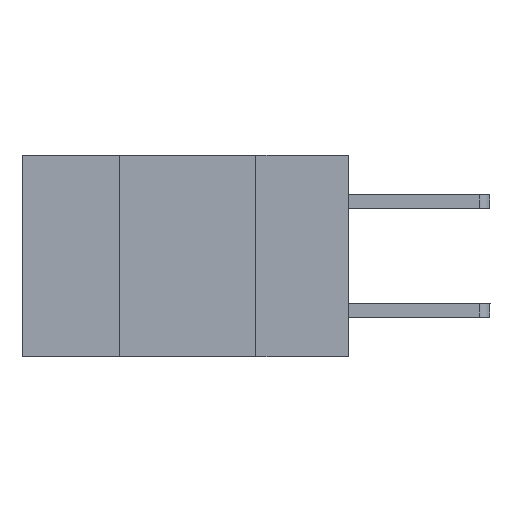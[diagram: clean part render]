
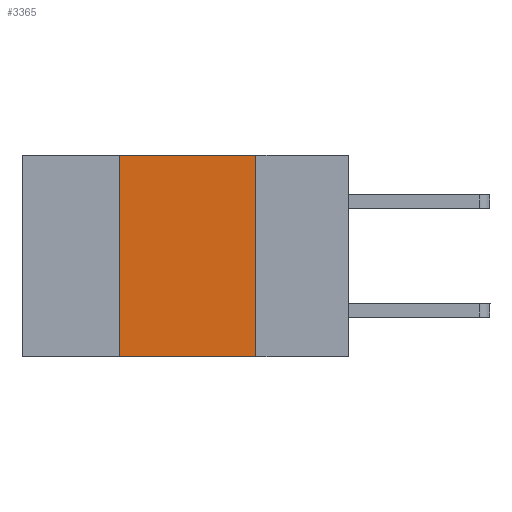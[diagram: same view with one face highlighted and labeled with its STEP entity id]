
A CAD part, left-side view. The second image highlights one B-rep face of the part: STEP entity #3365.
In plain terms, the highlighted planar face has unit normal (-1, 0, 0).
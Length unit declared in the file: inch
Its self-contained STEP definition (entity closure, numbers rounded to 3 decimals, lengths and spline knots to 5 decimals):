
#161 = VERTEX_POINT ( 'NONE', #2700 ) ;
#421 = ORIENTED_EDGE ( 'NONE', *, *, #1642, .T. ) ;
#592 = AXIS2_PLACEMENT_3D ( 'NONE', #3027, #1663, #1645 ) ;
#651 = EDGE_CURVE ( 'NONE', #161, #4681, #4739, .T. ) ;
#888 = EDGE_CURVE ( 'NONE', #4681, #3417, #6702, .T. ) ;
#996 = EDGE_CURVE ( 'NONE', #3417, #4597, #3637, .T. ) ;
#1642 = EDGE_CURVE ( 'NONE', #161, #4597, #7716, .T. ) ;
#1645 = DIRECTION ( 'NONE',  ( 0., 0., -1. ) ) ;
#1663 = DIRECTION ( 'NONE',  ( 1., 0., 0. ) ) ;
#1760 = PLANE ( 'NONE',  #592 ) ;
#2589 = ORIENTED_EDGE ( 'NONE', *, *, #888, .F. ) ;
#2700 = CARTESIAN_POINT ( 'NONE',  ( 0., 0.42, -0.37 ) ) ;
#3027 = CARTESIAN_POINT ( 'NONE',  ( 0., 0.6, 0. ) ) ;
#3066 = DIRECTION ( 'NONE',  ( 0., -1., 0. ) ) ;
#3162 = DIRECTION ( 'NONE',  ( 0., -1., 0. ) ) ;
#3365 = ADVANCED_FACE ( 'NONE', ( #3757 ), #1760, .F. ) ;
#3417 = VERTEX_POINT ( 'NONE', #8166 ) ;
#3637 = LINE ( 'NONE', #5191, #5474 ) ;
#3757 = FACE_OUTER_BOUND ( 'NONE', #5727, .T. ) ;
#4597 = VERTEX_POINT ( 'NONE', #7343 ) ;
#4681 = VERTEX_POINT ( 'NONE', #6248 ) ;
#4739 = LINE ( 'NONE', #7627, #9024 ) ;
#4929 = VECTOR ( 'NONE', #3162, 39.37008 ) ;
#5191 = CARTESIAN_POINT ( 'NONE',  ( 0., 0.17, -0.37 ) ) ;
#5474 = VECTOR ( 'NONE', #8913, 39.37008 ) ;
#5727 = EDGE_LOOP ( 'NONE', ( #6177, #2589, #6173, #421 ) ) ;
#5986 = VECTOR ( 'NONE', #3066, 39.37008 ) ;
#6173 = ORIENTED_EDGE ( 'NONE', *, *, #651, .F. ) ;
#6177 = ORIENTED_EDGE ( 'NONE', *, *, #996, .F. ) ;
#6248 = CARTESIAN_POINT ( 'NONE',  ( 0., 0.42, 0. ) ) ;
#6702 = LINE ( 'NONE', #7554, #4929 ) ;
#6846 = CARTESIAN_POINT ( 'NONE',  ( 0., 0.6, -0.37 ) ) ;
#7343 = CARTESIAN_POINT ( 'NONE',  ( 0., 0.17, -0.37 ) ) ;
#7554 = CARTESIAN_POINT ( 'NONE',  ( 0., 0.6, 0. ) ) ;
#7627 = CARTESIAN_POINT ( 'NONE',  ( 0., 0.42, -0.37 ) ) ;
#7716 = LINE ( 'NONE', #6846, #5986 ) ;
#8043 = DIRECTION ( 'NONE',  ( 0., 0., 1. ) ) ;
#8166 = CARTESIAN_POINT ( 'NONE',  ( 0., 0.17, 0. ) ) ;
#8913 = DIRECTION ( 'NONE',  ( 0., 0., -1. ) ) ;
#9024 = VECTOR ( 'NONE', #8043, 39.37008 ) ;
